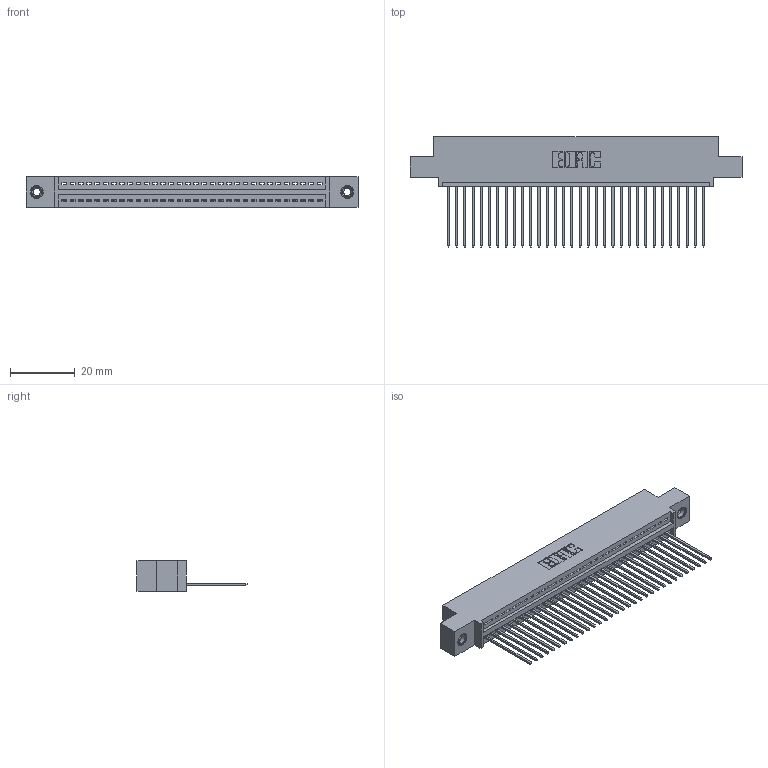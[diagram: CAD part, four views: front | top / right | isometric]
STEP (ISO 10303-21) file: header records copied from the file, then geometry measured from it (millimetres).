
FILE_DESCRIPTION (( 'STEP AP203' ), '1' );
FILE_NAME ('345-032-541-408.STEP', '2018-08-24T07:04:22', ( '' ), ( '' ), 'SwSTEP 2.0', 'SolidWorks 2016', '' );
FILE_SCHEMA (( 'CONFIG_CONTROL_DESIGN' ));
Length unit declared in the file: inch
Products named in the file (4): 345-292-001_345-293-141; 345-250-001_345-250-003-102; 345-032-541-408; 345 Part_0.110 Offset - 0.156 Dia-TI
Assembly tree (35 placements, depth 2):
  345-032-541-408
    345 Part_0.110 Offset - 0.156 Dia-TI
    345-292-001_345-293-141  x32
    345-250-001_345-250-003-102  x2
Bounding box: 102.49 x 33.96 x 9.4 mm (x, y, z)
Volume: 9678.3 mm3; surface area: 13448 mm2
Topology: 35 solids, 35 shells, 2046 faces, 6121 edges, 4030 vertices
Faces by surface type: plane 1396, cylinder 634, cone 12, torus 4
Entity records: 26766 total; most frequent: CARTESIAN_POINT 4619, ORIENTED_EDGE 4578, DIRECTION 4075, EDGE_CURVE 2289, VECTOR 2009, LINE 2009, VERTEX_POINT 1520, AXIS2_PLACEMENT_3D 1033
